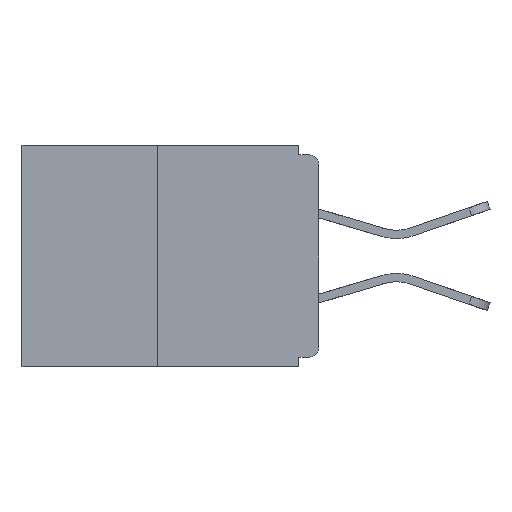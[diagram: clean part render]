
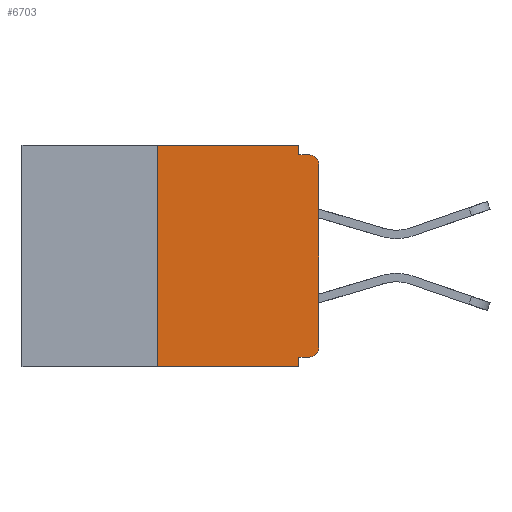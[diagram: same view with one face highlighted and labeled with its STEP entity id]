
A CAD part, left-side view. The second image highlights one B-rep face of the part: STEP entity #6703.
In plain terms, the highlighted planar face has unit normal (-1, 0, 0).
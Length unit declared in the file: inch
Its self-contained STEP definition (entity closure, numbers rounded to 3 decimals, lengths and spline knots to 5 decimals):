
#35 = AXIS2_PLACEMENT_3D ( 'NONE', #7297, #7979, #11353 ) ;
#332 = ORIENTED_EDGE ( 'NONE', *, *, #11977, .F. ) ;
#339 = EDGE_CURVE ( 'NONE', #10025, #5449, #871, .T. ) ;
#678 = VECTOR ( 'NONE', #10291, 39.37008 ) ;
#871 = CIRCLE ( 'NONE', #9845, 0.015 ) ;
#1370 = LINE ( 'NONE', #9342, #6283 ) ;
#1440 = EDGE_CURVE ( 'NONE', #6659, #5449, #6801, .T. ) ;
#1491 = EDGE_CURVE ( 'NONE', #6911, #11852, #8359, .T. ) ;
#1832 = DIRECTION ( 'NONE',  ( 0., -1., 0. ) ) ;
#1915 = EDGE_CURVE ( 'NONE', #5146, #12323, #11884, .T. ) ;
#1923 = VERTEX_POINT ( 'NONE', #10181 ) ;
#1981 = DIRECTION ( 'NONE',  ( 0., -1., 0. ) ) ;
#2056 = EDGE_CURVE ( 'NONE', #11852, #6659, #8148, .T. ) ;
#2332 = ORIENTED_EDGE ( 'NONE', *, *, #1915, .T. ) ;
#2377 = CARTESIAN_POINT ( 'NONE',  ( 0., 0.031, -0.343 ) ) ;
#2707 = EDGE_LOOP ( 'NONE', ( #5247, #8361, #9312, #332, #9117, #2332, #6847, #3846, #4483, #9319 ) ) ;
#3076 = CARTESIAN_POINT ( 'NONE',  ( 0., 0.015, -0.328 ) ) ;
#3205 = CARTESIAN_POINT ( 'NONE',  ( 0., 0.46, 0. ) ) ;
#3648 = CARTESIAN_POINT ( 'NONE',  ( 0., 0.25, 0. ) ) ;
#3846 = ORIENTED_EDGE ( 'NONE', *, *, #339, .T. ) ;
#4199 = DIRECTION ( 'NONE',  ( -1., 0., 0. ) ) ;
#4229 = VECTOR ( 'NONE', #7374, 39.37008 ) ;
#4232 = DIRECTION ( 'NONE',  ( 0., 0., -1. ) ) ;
#4315 = CARTESIAN_POINT ( 'NONE',  ( 0., 0., -0.313 ) ) ;
#4483 = ORIENTED_EDGE ( 'NONE', *, *, #1440, .F. ) ;
#4518 = CARTESIAN_POINT ( 'NONE',  ( 0., 0.031, 0. ) ) ;
#4698 = CARTESIAN_POINT ( 'NONE',  ( 0., 0.015, -0.015 ) ) ;
#4744 = LINE ( 'NONE', #3648, #8177 ) ;
#5115 = VECTOR ( 'NONE', #12215, 39.37008 ) ;
#5146 = VERTEX_POINT ( 'NONE', #3076 ) ;
#5234 = CARTESIAN_POINT ( 'NONE',  ( 0., 0.031, -0.328 ) ) ;
#5247 = ORIENTED_EDGE ( 'NONE', *, *, #1491, .F. ) ;
#5449 = VERTEX_POINT ( 'NONE', #4698 ) ;
#5601 = CARTESIAN_POINT ( 'NONE',  ( 0., 0.031, 0. ) ) ;
#5651 = EDGE_CURVE ( 'NONE', #5146, #10230, #1370, .T. ) ;
#5894 = CARTESIAN_POINT ( 'NONE',  ( 0., 0., -0.03 ) ) ;
#5912 = LINE ( 'NONE', #8455, #678 ) ;
#6060 = CARTESIAN_POINT ( 'NONE',  ( 0., 0.015, -0.313 ) ) ;
#6192 = DIRECTION ( 'NONE',  ( -1., 0., 0. ) ) ;
#6283 = VECTOR ( 'NONE', #12330, 39.37008 ) ;
#6365 = DIRECTION ( 'NONE',  ( 0., 0., -1. ) ) ;
#6494 = VECTOR ( 'NONE', #6365, 39.37008 ) ;
#6659 = VERTEX_POINT ( 'NONE', #12481 ) ;
#6703 = ADVANCED_FACE ( 'NONE', ( #10990 ), #10320, .F. ) ;
#6801 = LINE ( 'NONE', #10788, #10757 ) ;
#6847 = ORIENTED_EDGE ( 'NONE', *, *, #11824, .T. ) ;
#6911 = VERTEX_POINT ( 'NONE', #9325 ) ;
#6942 = LINE ( 'NONE', #7012, #11909 ) ;
#7012 = CARTESIAN_POINT ( 'NONE',  ( 0., 0.46, -0.343 ) ) ;
#7297 = CARTESIAN_POINT ( 'NONE',  ( 0., 0.46, 0. ) ) ;
#7374 = DIRECTION ( 'NONE',  ( 0., 0., -1. ) ) ;
#7761 = DIRECTION ( 'NONE',  ( 0., 0., 1. ) ) ;
#7979 = DIRECTION ( 'NONE',  ( 1., 0., 0. ) ) ;
#8148 = LINE ( 'NONE', #5601, #4229 ) ;
#8177 = VECTOR ( 'NONE', #7761, 39.37008 ) ;
#8359 = LINE ( 'NONE', #3205, #5115 ) ;
#8361 = ORIENTED_EDGE ( 'NONE', *, *, #12887, .F. ) ;
#8455 = CARTESIAN_POINT ( 'NONE',  ( 0., 0., 0. ) ) ;
#8743 = VERTEX_POINT ( 'NONE', #9624 ) ;
#9095 = AXIS2_PLACEMENT_3D ( 'NONE', #6060, #6192, #4232 ) ;
#9117 = ORIENTED_EDGE ( 'NONE', *, *, #5651, .F. ) ;
#9312 = ORIENTED_EDGE ( 'NONE', *, *, #12136, .T. ) ;
#9319 = ORIENTED_EDGE ( 'NONE', *, *, #2056, .F. ) ;
#9325 = CARTESIAN_POINT ( 'NONE',  ( 0., 0.25, 0. ) ) ;
#9342 = CARTESIAN_POINT ( 'NONE',  ( 0., 0., -0.328 ) ) ;
#9624 = CARTESIAN_POINT ( 'NONE',  ( 0., 0.25, -0.343 ) ) ;
#9845 = AXIS2_PLACEMENT_3D ( 'NONE', #12301, #4199, #12184 ) ;
#10025 = VERTEX_POINT ( 'NONE', #5894 ) ;
#10181 = CARTESIAN_POINT ( 'NONE',  ( 0., 0.031, -0.343 ) ) ;
#10230 = VERTEX_POINT ( 'NONE', #5234 ) ;
#10291 = DIRECTION ( 'NONE',  ( 0., 0., 1. ) ) ;
#10320 = PLANE ( 'NONE',  #35 ) ;
#10757 = VECTOR ( 'NONE', #1832, 39.37008 ) ;
#10788 = CARTESIAN_POINT ( 'NONE',  ( 0., 0., -0.015 ) ) ;
#10990 = FACE_OUTER_BOUND ( 'NONE', #2707, .T. ) ;
#11327 = LINE ( 'NONE', #2377, #6494 ) ;
#11353 = DIRECTION ( 'NONE',  ( 0., 0., -1. ) ) ;
#11824 = EDGE_CURVE ( 'NONE', #12323, #10025, #5912, .T. ) ;
#11852 = VERTEX_POINT ( 'NONE', #4518 ) ;
#11884 = CIRCLE ( 'NONE', #9095, 0.015 ) ;
#11909 = VECTOR ( 'NONE', #1981, 39.37008 ) ;
#11977 = EDGE_CURVE ( 'NONE', #10230, #1923, #11327, .T. ) ;
#12136 = EDGE_CURVE ( 'NONE', #8743, #1923, #6942, .T. ) ;
#12184 = DIRECTION ( 'NONE',  ( 0., 0., -1. ) ) ;
#12215 = DIRECTION ( 'NONE',  ( 0., -1., 0. ) ) ;
#12301 = CARTESIAN_POINT ( 'NONE',  ( 0., 0.015, -0.03 ) ) ;
#12323 = VERTEX_POINT ( 'NONE', #4315 ) ;
#12330 = DIRECTION ( 'NONE',  ( 0., 1., 0. ) ) ;
#12481 = CARTESIAN_POINT ( 'NONE',  ( 0., 0.031, -0.015 ) ) ;
#12887 = EDGE_CURVE ( 'NONE', #8743, #6911, #4744, .T. ) ;
